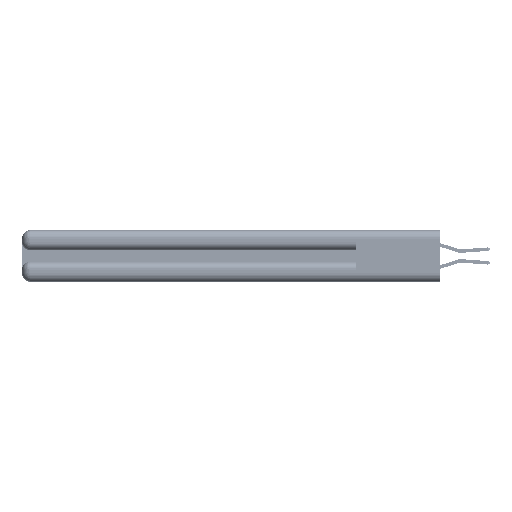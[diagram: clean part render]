
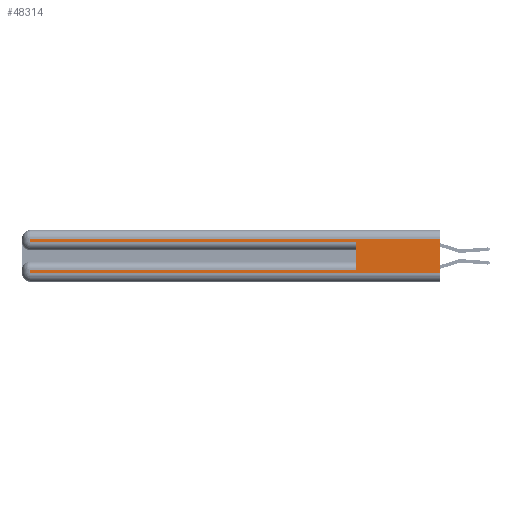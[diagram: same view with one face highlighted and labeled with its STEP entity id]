
A CAD part, left-side view. The second image highlights one B-rep face of the part: STEP entity #48314.
In plain terms, the highlighted planar face has unit normal (-1, 0, 0).
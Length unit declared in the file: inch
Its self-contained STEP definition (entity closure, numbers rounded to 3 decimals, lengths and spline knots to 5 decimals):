
#2177 = DIRECTION ( 'NONE',  ( 0., 0., -1. ) ) ;
#2407 = LINE ( 'NONE', #36752, #25159 ) ;
#2627 = CARTESIAN_POINT ( 'NONE',  ( 0., 0., 0.31 ) ) ;
#2867 = ORIENTED_EDGE ( 'NONE', *, *, #32075, .F. ) ;
#3006 = CARTESIAN_POINT ( 'NONE',  ( 0., 0.6, 0.085 ) ) ;
#4832 = CARTESIAN_POINT ( 'NONE',  ( 0., 0., 0.285 ) ) ;
#6402 = ORIENTED_EDGE ( 'NONE', *, *, #42153, .T. ) ;
#7266 = ORIENTED_EDGE ( 'NONE', *, *, #24606, .F. ) ;
#8437 = PLANE ( 'NONE',  #26151 ) ;
#8778 = VERTEX_POINT ( 'NONE', #31081 ) ;
#10316 = DIRECTION ( 'NONE',  ( 0., 0., 1. ) ) ;
#11058 = CARTESIAN_POINT ( 'NONE',  ( 0., 2.94, 0.285 ) ) ;
#12260 = DIRECTION ( 'NONE',  ( 0., 0., -1. ) ) ;
#12821 = LINE ( 'NONE', #27631, #51206 ) ;
#13409 = CARTESIAN_POINT ( 'NONE',  ( 0., 2.94, 0.085 ) ) ;
#13628 = EDGE_LOOP ( 'NONE', ( #7266, #23618, #43280, #31927, #2867, #26214, #6402, #52298 ) ) ;
#15666 = LINE ( 'NONE', #45779, #18293 ) ;
#16829 = CARTESIAN_POINT ( 'NONE',  ( 0., 2.94, 0.06 ) ) ;
#18053 = CARTESIAN_POINT ( 'NONE',  ( 0., 0.6, 0.285 ) ) ;
#18293 = VECTOR ( 'NONE', #29211, 39.37008 ) ;
#19859 = VERTEX_POINT ( 'NONE', #13409 ) ;
#19974 = CARTESIAN_POINT ( 'NONE',  ( 0., 0., 0.06 ) ) ;
#20625 = CARTESIAN_POINT ( 'NONE',  ( 0., 0., 0.31 ) ) ;
#21423 = LINE ( 'NONE', #40328, #31864 ) ;
#21661 = EDGE_CURVE ( 'NONE', #21773, #19859, #21423, .T. ) ;
#21773 = VERTEX_POINT ( 'NONE', #3006 ) ;
#23618 = ORIENTED_EDGE ( 'NONE', *, *, #28910, .T. ) ;
#23716 = DIRECTION ( 'NONE',  ( 0., 1., 0. ) ) ;
#24606 = EDGE_CURVE ( 'NONE', #36369, #45648, #12821, .T. ) ;
#25159 = VECTOR ( 'NONE', #45089, 39.37008 ) ;
#25216 = CARTESIAN_POINT ( 'NONE',  ( 0., 0., 0.06 ) ) ;
#25507 = VECTOR ( 'NONE', #10316, 39.37008 ) ;
#26151 = AXIS2_PLACEMENT_3D ( 'NONE', #45755, #28829, #12260 ) ;
#26214 = ORIENTED_EDGE ( 'NONE', *, *, #21661, .T. ) ;
#26554 = VECTOR ( 'NONE', #29412, 39.37008 ) ;
#26822 = LINE ( 'NONE', #2627, #28738 ) ;
#27631 = CARTESIAN_POINT ( 'NONE',  ( 0., 0., 0.37 ) ) ;
#27803 = VERTEX_POINT ( 'NONE', #11058 ) ;
#28271 = DIRECTION ( 'NONE',  ( 0., 1., 0. ) ) ;
#28738 = VECTOR ( 'NONE', #23716, 39.37008 ) ;
#28829 = DIRECTION ( 'NONE',  ( 1., 0., 0. ) ) ;
#28849 = VECTOR ( 'NONE', #52941, 39.37008 ) ;
#28910 = EDGE_CURVE ( 'NONE', #36369, #8778, #26822, .T. ) ;
#29211 = DIRECTION ( 'NONE',  ( 0., 0., -1. ) ) ;
#29412 = DIRECTION ( 'NONE',  ( 0., -1., 0. ) ) ;
#31081 = CARTESIAN_POINT ( 'NONE',  ( 0., 2.94, 0.31 ) ) ;
#31575 = EDGE_CURVE ( 'NONE', #40851, #45648, #33441, .T. ) ;
#31864 = VECTOR ( 'NONE', #28271, 39.37008 ) ;
#31927 = ORIENTED_EDGE ( 'NONE', *, *, #51376, .T. ) ;
#32075 = EDGE_CURVE ( 'NONE', #21773, #36509, #32716, .T. ) ;
#32451 = EDGE_CURVE ( 'NONE', #8778, #27803, #15666, .T. ) ;
#32716 = LINE ( 'NONE', #35299, #25507 ) ;
#33441 = LINE ( 'NONE', #19974, #28849 ) ;
#35299 = CARTESIAN_POINT ( 'NONE',  ( 0., 0.6, 0.145 ) ) ;
#36369 = VERTEX_POINT ( 'NONE', #20625 ) ;
#36509 = VERTEX_POINT ( 'NONE', #18053 ) ;
#36531 = FACE_OUTER_BOUND ( 'NONE', #13628, .T. ) ;
#36752 = CARTESIAN_POINT ( 'NONE',  ( 0., 2.94, 0.37 ) ) ;
#40328 = CARTESIAN_POINT ( 'NONE',  ( 0., 0., 0.085 ) ) ;
#40851 = VERTEX_POINT ( 'NONE', #16829 ) ;
#42153 = EDGE_CURVE ( 'NONE', #19859, #40851, #2407, .T. ) ;
#43280 = ORIENTED_EDGE ( 'NONE', *, *, #32451, .T. ) ;
#45089 = DIRECTION ( 'NONE',  ( 0., 0., -1. ) ) ;
#45648 = VERTEX_POINT ( 'NONE', #25216 ) ;
#45755 = CARTESIAN_POINT ( 'NONE',  ( 0., 0., 0.37 ) ) ;
#45779 = CARTESIAN_POINT ( 'NONE',  ( 0., 2.94, 0.37 ) ) ;
#48314 = ADVANCED_FACE ( 'NONE', ( #36531 ), #8437, .F. ) ;
#48691 = LINE ( 'NONE', #4832, #26554 ) ;
#51206 = VECTOR ( 'NONE', #2177, 39.37008 ) ;
#51376 = EDGE_CURVE ( 'NONE', #27803, #36509, #48691, .T. ) ;
#52298 = ORIENTED_EDGE ( 'NONE', *, *, #31575, .T. ) ;
#52941 = DIRECTION ( 'NONE',  ( 0., -1., 0. ) ) ;
